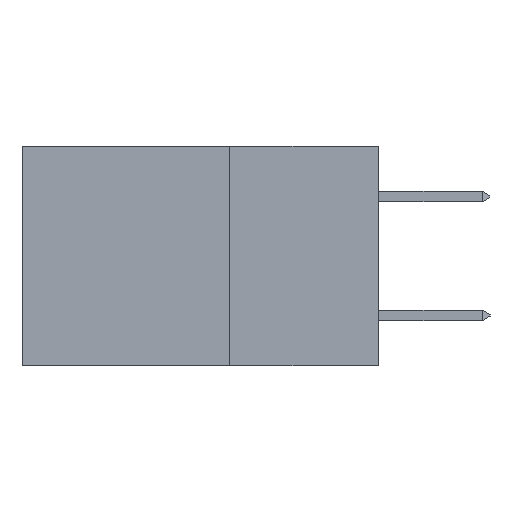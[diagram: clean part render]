
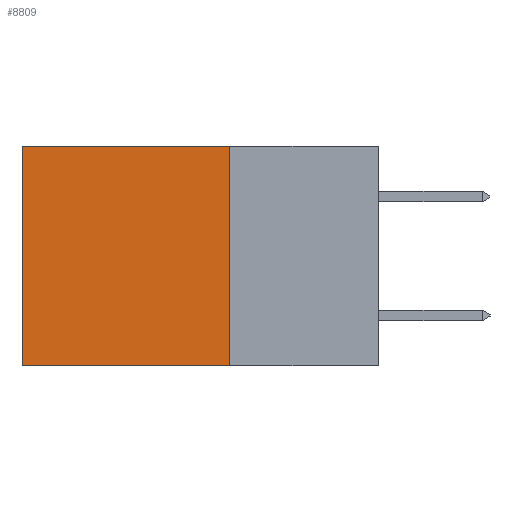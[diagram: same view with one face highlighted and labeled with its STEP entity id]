
A CAD part, left-side view. The second image highlights one B-rep face of the part: STEP entity #8809.
In plain terms, the highlighted planar face has unit normal (-1, 0, 0).
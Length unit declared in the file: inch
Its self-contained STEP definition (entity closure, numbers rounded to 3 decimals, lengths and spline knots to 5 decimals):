
#175 = VERTEX_POINT ( 'NONE', #17791 ) ;
#616 = EDGE_CURVE ( 'NONE', #4598, #807, #3366, .T. ) ;
#807 = VERTEX_POINT ( 'NONE', #19057 ) ;
#962 = PLANE ( 'NONE',  #17929 ) ;
#2480 = DIRECTION ( 'NONE',  ( 0., 0., -1. ) ) ;
#2988 = VECTOR ( 'NONE', #7809, 39.37008 ) ;
#3366 = LINE ( 'NONE', #5705, #18532 ) ;
#3611 = VECTOR ( 'NONE', #18134, 39.37008 ) ;
#4082 = LINE ( 'NONE', #18201, #3611 ) ;
#4466 = LINE ( 'NONE', #12996, #11842 ) ;
#4598 = VERTEX_POINT ( 'NONE', #7708 ) ;
#5705 = CARTESIAN_POINT ( 'NONE',  ( 0.2615, 0.25, -0.37 ) ) ;
#5928 = VERTEX_POINT ( 'NONE', #9223 ) ;
#5994 = EDGE_CURVE ( 'NONE', #4598, #175, #6965, .T. ) ;
#6965 = LINE ( 'NONE', #7385, #2988 ) ;
#7385 = CARTESIAN_POINT ( 'NONE',  ( 0.2615, 0.25, 0. ) ) ;
#7419 = EDGE_CURVE ( 'NONE', #175, #5928, #4082, .T. ) ;
#7708 = CARTESIAN_POINT ( 'NONE',  ( 0.2615, 0.25, 0. ) ) ;
#7809 = DIRECTION ( 'NONE',  ( 0., 1., 0. ) ) ;
#8312 = FACE_OUTER_BOUND ( 'NONE', #12809, .T. ) ;
#8671 = DIRECTION ( 'NONE',  ( 0., 1., 0. ) ) ;
#8809 = ADVANCED_FACE ( 'NONE', ( #8312 ), #962, .F. ) ;
#9175 = ORIENTED_EDGE ( 'NONE', *, *, #12900, .F. ) ;
#9223 = CARTESIAN_POINT ( 'NONE',  ( 0.2615, 0.6, -0.37 ) ) ;
#11345 = DIRECTION ( 'NONE',  ( 1., 0., 0. ) ) ;
#11515 = ORIENTED_EDGE ( 'NONE', *, *, #7419, .T. ) ;
#11842 = VECTOR ( 'NONE', #8671, 39.37008 ) ;
#12809 = EDGE_LOOP ( 'NONE', ( #11515, #9175, #18658, #14172 ) ) ;
#12900 = EDGE_CURVE ( 'NONE', #807, #5928, #4466, .T. ) ;
#12996 = CARTESIAN_POINT ( 'NONE',  ( 0.2615, 0.25, -0.37 ) ) ;
#14101 = DIRECTION ( 'NONE',  ( 0., 0., -1. ) ) ;
#14172 = ORIENTED_EDGE ( 'NONE', *, *, #5994, .T. ) ;
#17791 = CARTESIAN_POINT ( 'NONE',  ( 0.2615, 0.6, 0. ) ) ;
#17929 = AXIS2_PLACEMENT_3D ( 'NONE', #18634, #11345, #2480 ) ;
#18134 = DIRECTION ( 'NONE',  ( 0., 0., -1. ) ) ;
#18201 = CARTESIAN_POINT ( 'NONE',  ( 0.2615, 0.6, -0.37 ) ) ;
#18532 = VECTOR ( 'NONE', #14101, 39.37008 ) ;
#18634 = CARTESIAN_POINT ( 'NONE',  ( 0.2615, 0.25, -0.37 ) ) ;
#18658 = ORIENTED_EDGE ( 'NONE', *, *, #616, .F. ) ;
#19057 = CARTESIAN_POINT ( 'NONE',  ( 0.2615, 0.25, -0.37 ) ) ;
